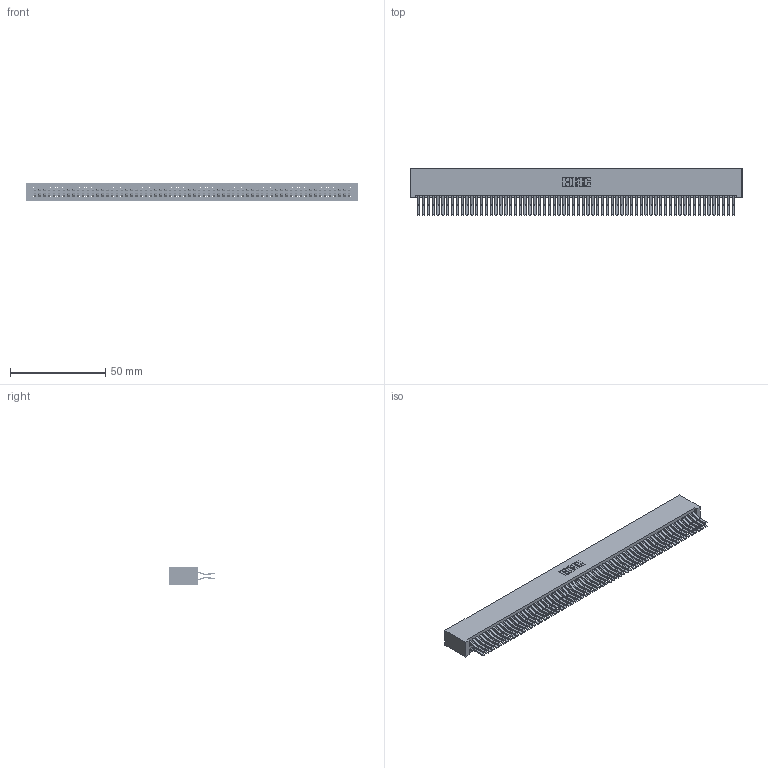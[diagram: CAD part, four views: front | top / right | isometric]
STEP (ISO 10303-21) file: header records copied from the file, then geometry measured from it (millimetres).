
FILE_DESCRIPTION (( 'STEP AP203' ), '1' );
FILE_NAME ('345-132-560-201.STEP', '2019-11-07T23:28:39', ( '' ), ( '' ), 'SwSTEP 2.0', 'SolidWorks 2016', '' );
FILE_SCHEMA (( 'CONFIG_CONTROL_DESIGN' ));
Length unit declared in the file: inch
Products named in the file (3): 345-292-001_560 Tail; 345-132-560-201; 345 Part_No Mounting Lugs
Assembly tree (133 placements, depth 2):
  345-132-560-201
    345 Part_No Mounting Lugs
    345-292-001_560 Tail  x132
Bounding box: 174.24 x 24.45 x 9.4 mm (x, y, z)
Volume: 18630.1 mm3; surface area: 30531.8 mm2
Topology: 133 solids, 133 shells, 6982 faces, 20777 edges, 13674 vertices
Faces by surface type: plane 4432, cylinder 2550
Entity records: 48365 total; most frequent: CARTESIAN_POINT 8084, ORIENTED_EDGE 8018, DIRECTION 7097, EDGE_CURVE 4009, VECTOR 3617, LINE 3617, VERTEX_POINT 2670, AXIS2_PLACEMENT_3D 1740
